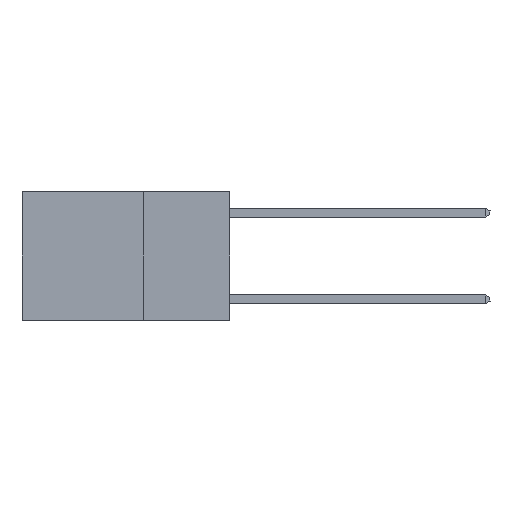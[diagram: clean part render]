
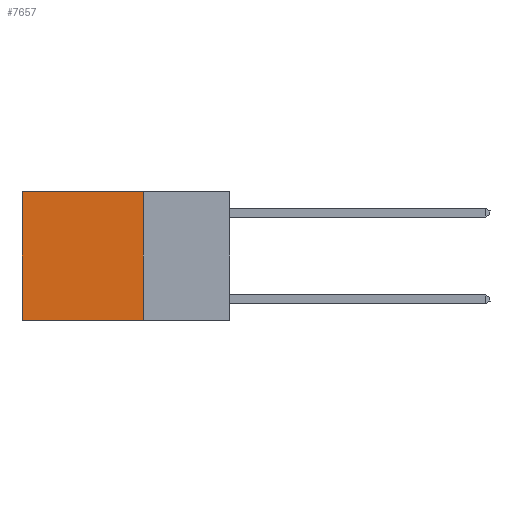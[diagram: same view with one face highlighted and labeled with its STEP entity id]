
A CAD part, left-side view. The second image highlights one B-rep face of the part: STEP entity #7657.
In plain terms, the highlighted planar face has unit normal (-1, 0, 0).
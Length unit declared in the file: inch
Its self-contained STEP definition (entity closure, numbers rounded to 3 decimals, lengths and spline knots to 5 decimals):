
#642 = VECTOR ( 'NONE', #13357, 39.37008 ) ;
#1407 = LINE ( 'NONE', #6027, #1526 ) ;
#1526 = VECTOR ( 'NONE', #10635, 39.37008 ) ;
#2081 = DIRECTION ( 'NONE',  ( 0., 1., 0. ) ) ;
#2523 = FACE_OUTER_BOUND ( 'NONE', #14269, .T. ) ;
#2801 = CARTESIAN_POINT ( 'NONE',  ( 0.2625, 0.6, 0. ) ) ;
#3467 = VECTOR ( 'NONE', #2081, 39.37008 ) ;
#3575 = ORIENTED_EDGE ( 'NONE', *, *, #14031, .F. ) ;
#3579 = EDGE_CURVE ( 'NONE', #11294, #12798, #5441, .T. ) ;
#3624 = CARTESIAN_POINT ( 'NONE',  ( 0.2625, 0.25, -0.37 ) ) ;
#3654 = DIRECTION ( 'NONE',  ( 0., 0., -1. ) ) ;
#4029 = AXIS2_PLACEMENT_3D ( 'NONE', #12927, #8491, #3654 ) ;
#4055 = LINE ( 'NONE', #12964, #7088 ) ;
#4922 = VERTEX_POINT ( 'NONE', #3624 ) ;
#5110 = DIRECTION ( 'NONE',  ( 0., 1., 0. ) ) ;
#5441 = LINE ( 'NONE', #8774, #642 ) ;
#6027 = CARTESIAN_POINT ( 'NONE',  ( 0.2625, 0.25, 0. ) ) ;
#7088 = VECTOR ( 'NONE', #5110, 39.37008 ) ;
#7657 = ADVANCED_FACE ( 'NONE', ( #2523 ), #13077, .F. ) ;
#7827 = CARTESIAN_POINT ( 'NONE',  ( 0.2625, 0.25, -0.37 ) ) ;
#7903 = CARTESIAN_POINT ( 'NONE',  ( 0.2625, 0.6, -0.37 ) ) ;
#8491 = DIRECTION ( 'NONE',  ( 1., 0., 0. ) ) ;
#8774 = CARTESIAN_POINT ( 'NONE',  ( 0.2625, 0.6, 0. ) ) ;
#9416 = CARTESIAN_POINT ( 'NONE',  ( 0.2625, 0.25, 0. ) ) ;
#9434 = ORIENTED_EDGE ( 'NONE', *, *, #3579, .T. ) ;
#10635 = DIRECTION ( 'NONE',  ( 0., 0., -1. ) ) ;
#11294 = VERTEX_POINT ( 'NONE', #2801 ) ;
#12512 = ORIENTED_EDGE ( 'NONE', *, *, #13956, .F. ) ;
#12798 = VERTEX_POINT ( 'NONE', #7903 ) ;
#12927 = CARTESIAN_POINT ( 'NONE',  ( 0.2625, 0.25, 0. ) ) ;
#12964 = CARTESIAN_POINT ( 'NONE',  ( 0.2625, 0.25, 0. ) ) ;
#13077 = PLANE ( 'NONE',  #4029 ) ;
#13328 = LINE ( 'NONE', #7827, #3467 ) ;
#13357 = DIRECTION ( 'NONE',  ( 0., 0., -1. ) ) ;
#13887 = EDGE_CURVE ( 'NONE', #14142, #11294, #4055, .T. ) ;
#13956 = EDGE_CURVE ( 'NONE', #14142, #4922, #1407, .T. ) ;
#14031 = EDGE_CURVE ( 'NONE', #4922, #12798, #13328, .T. ) ;
#14142 = VERTEX_POINT ( 'NONE', #9416 ) ;
#14269 = EDGE_LOOP ( 'NONE', ( #9434, #3575, #12512, #14574 ) ) ;
#14574 = ORIENTED_EDGE ( 'NONE', *, *, #13887, .T. ) ;
